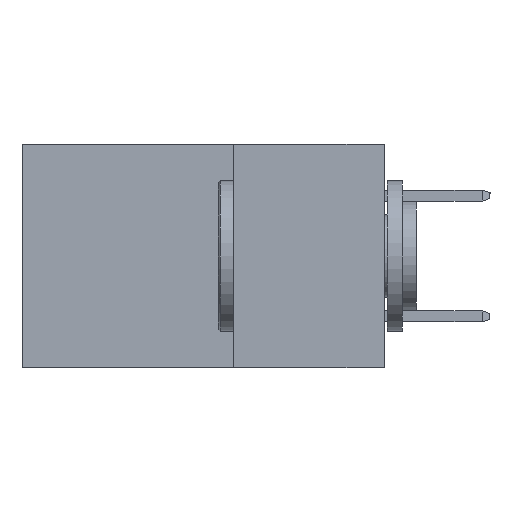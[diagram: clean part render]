
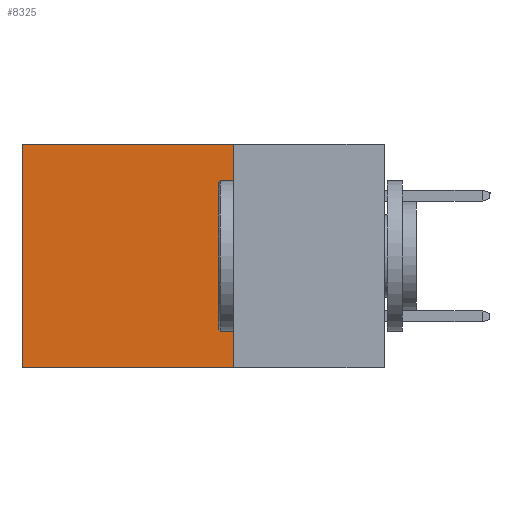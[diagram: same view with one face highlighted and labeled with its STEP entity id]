
A CAD part, left-side view. The second image highlights one B-rep face of the part: STEP entity #8325.
In plain terms, the highlighted planar face has unit normal (-1, 0, 0).
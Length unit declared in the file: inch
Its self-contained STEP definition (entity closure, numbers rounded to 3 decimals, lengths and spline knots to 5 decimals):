
#1326 = VECTOR ( 'NONE', #14075, 39.37008 ) ;
#2507 = VERTEX_POINT ( 'NONE', #9022 ) ;
#4595 = AXIS2_PLACEMENT_3D ( 'NONE', #15367, #12598, #12403 ) ;
#5337 = VECTOR ( 'NONE', #13859, 39.37008 ) ;
#5785 = CARTESIAN_POINT ( 'NONE',  ( 0.2615, 0.6, -0.37 ) ) ;
#6187 = VERTEX_POINT ( 'NONE', #18731 ) ;
#6188 = PLANE ( 'NONE',  #4595 ) ;
#6326 = CARTESIAN_POINT ( 'NONE',  ( 0.2615, 0.6, 0. ) ) ;
#6618 = ORIENTED_EDGE ( 'NONE', *, *, #17376, .F. ) ;
#6649 = LINE ( 'NONE', #6940, #18669 ) ;
#6940 = CARTESIAN_POINT ( 'NONE',  ( 0.2615, 0.25, 0. ) ) ;
#7295 = VECTOR ( 'NONE', #7357, 39.37008 ) ;
#7357 = DIRECTION ( 'NONE',  ( 0., 1., 0. ) ) ;
#8325 = ADVANCED_FACE ( 'NONE', ( #15465 ), #6188, .F. ) ;
#9022 = CARTESIAN_POINT ( 'NONE',  ( 0.2615, 0.25, -0.37 ) ) ;
#9294 = ORIENTED_EDGE ( 'NONE', *, *, #10577, .F. ) ;
#10263 = EDGE_LOOP ( 'NONE', ( #12329, #6618, #9294, #13182 ) ) ;
#10577 = EDGE_CURVE ( 'NONE', #6187, #2507, #12355, .T. ) ;
#10589 = VERTEX_POINT ( 'NONE', #6326 ) ;
#11377 = VERTEX_POINT ( 'NONE', #5785 ) ;
#12002 = CARTESIAN_POINT ( 'NONE',  ( 0.2615, 0.25, -0.37 ) ) ;
#12329 = ORIENTED_EDGE ( 'NONE', *, *, #14225, .T. ) ;
#12355 = LINE ( 'NONE', #12002, #1326 ) ;
#12403 = DIRECTION ( 'NONE',  ( 0., 0., -1. ) ) ;
#12415 = LINE ( 'NONE', #15383, #5337 ) ;
#12598 = DIRECTION ( 'NONE',  ( 1., 0., 0. ) ) ;
#13182 = ORIENTED_EDGE ( 'NONE', *, *, #17245, .T. ) ;
#13679 = CARTESIAN_POINT ( 'NONE',  ( 0.2615, 0.25, -0.37 ) ) ;
#13859 = DIRECTION ( 'NONE',  ( 0., 0., -1. ) ) ;
#14075 = DIRECTION ( 'NONE',  ( 0., 0., -1. ) ) ;
#14225 = EDGE_CURVE ( 'NONE', #10589, #11377, #12415, .T. ) ;
#15203 = LINE ( 'NONE', #13679, #7295 ) ;
#15367 = CARTESIAN_POINT ( 'NONE',  ( 0.2615, 0.25, -0.37 ) ) ;
#15383 = CARTESIAN_POINT ( 'NONE',  ( 0.2615, 0.6, -0.37 ) ) ;
#15465 = FACE_OUTER_BOUND ( 'NONE', #10263, .T. ) ;
#17245 = EDGE_CURVE ( 'NONE', #6187, #10589, #6649, .T. ) ;
#17376 = EDGE_CURVE ( 'NONE', #2507, #11377, #15203, .T. ) ;
#17653 = DIRECTION ( 'NONE',  ( 0., 1., 0. ) ) ;
#18669 = VECTOR ( 'NONE', #17653, 39.37008 ) ;
#18731 = CARTESIAN_POINT ( 'NONE',  ( 0.2615, 0.25, 0. ) ) ;
